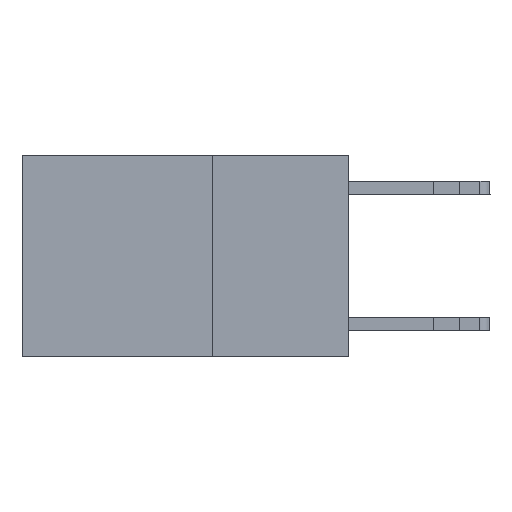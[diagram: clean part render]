
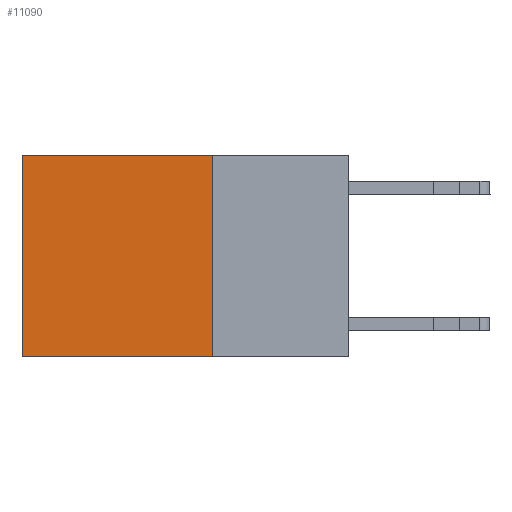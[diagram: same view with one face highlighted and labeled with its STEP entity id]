
A CAD part, left-side view. The second image highlights one B-rep face of the part: STEP entity #11090.
In plain terms, the highlighted planar face has unit normal (-1, 0, 0).
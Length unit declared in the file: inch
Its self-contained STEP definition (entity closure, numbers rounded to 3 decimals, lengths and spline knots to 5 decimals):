
#64 = DIRECTION ( 'NONE',  ( 0., 0., -1. ) ) ;
#91 = DIRECTION ( 'NONE',  ( 0., 0., -1. ) ) ;
#342 = DIRECTION ( 'NONE',  ( 1., 0., 0. ) ) ;
#380 = ORIENTED_EDGE ( 'NONE', *, *, #9923, .T. ) ;
#582 = CARTESIAN_POINT ( 'NONE',  ( 0.2625, 0.6, -0.37 ) ) ;
#602 = AXIS2_PLACEMENT_3D ( 'NONE', #10636, #342, #64 ) ;
#640 = CARTESIAN_POINT ( 'NONE',  ( 0.2625, 0.25, -0.37 ) ) ;
#783 = CARTESIAN_POINT ( 'NONE',  ( 0.2625, 0.25, 0. ) ) ;
#1365 = CARTESIAN_POINT ( 'NONE',  ( 0.2625, 0.25, 0. ) ) ;
#2021 = VERTEX_POINT ( 'NONE', #13042 ) ;
#2173 = ORIENTED_EDGE ( 'NONE', *, *, #9091, .T. ) ;
#2189 = DIRECTION ( 'NONE',  ( 0., 0., -1. ) ) ;
#3525 = VECTOR ( 'NONE', #5996, 39.37008 ) ;
#3553 = CARTESIAN_POINT ( 'NONE',  ( 0.2625, 0.25, 0. ) ) ;
#4829 = FACE_OUTER_BOUND ( 'NONE', #6822, .T. ) ;
#5447 = VECTOR ( 'NONE', #91, 39.37008 ) ;
#5620 = VERTEX_POINT ( 'NONE', #783 ) ;
#5996 = DIRECTION ( 'NONE',  ( 0., 1., 0. ) ) ;
#6046 = ORIENTED_EDGE ( 'NONE', *, *, #10484, .F. ) ;
#6157 = ORIENTED_EDGE ( 'NONE', *, *, #7837, .F. ) ;
#6822 = EDGE_LOOP ( 'NONE', ( #2173, #6157, #6046, #380 ) ) ;
#6999 = LINE ( 'NONE', #1365, #3525 ) ;
#7476 = DIRECTION ( 'NONE',  ( 0., 1., 0. ) ) ;
#7837 = EDGE_CURVE ( 'NONE', #11556, #13974, #10798, .T. ) ;
#9091 = EDGE_CURVE ( 'NONE', #2021, #13974, #10441, .T. ) ;
#9923 = EDGE_CURVE ( 'NONE', #5620, #2021, #6999, .T. ) ;
#10221 = CARTESIAN_POINT ( 'NONE',  ( 0.2625, 0.6, 0. ) ) ;
#10441 = LINE ( 'NONE', #10221, #5447 ) ;
#10484 = EDGE_CURVE ( 'NONE', #5620, #11556, #13929, .T. ) ;
#10636 = CARTESIAN_POINT ( 'NONE',  ( 0.2625, 0.25, 0. ) ) ;
#10798 = LINE ( 'NONE', #640, #12897 ) ;
#11003 = VECTOR ( 'NONE', #2189, 39.37008 ) ;
#11090 = ADVANCED_FACE ( 'NONE', ( #4829 ), #12679, .F. ) ;
#11556 = VERTEX_POINT ( 'NONE', #13949 ) ;
#12679 = PLANE ( 'NONE',  #602 ) ;
#12897 = VECTOR ( 'NONE', #7476, 39.37008 ) ;
#13042 = CARTESIAN_POINT ( 'NONE',  ( 0.2625, 0.6, 0. ) ) ;
#13929 = LINE ( 'NONE', #3553, #11003 ) ;
#13949 = CARTESIAN_POINT ( 'NONE',  ( 0.2625, 0.25, -0.37 ) ) ;
#13974 = VERTEX_POINT ( 'NONE', #582 ) ;
